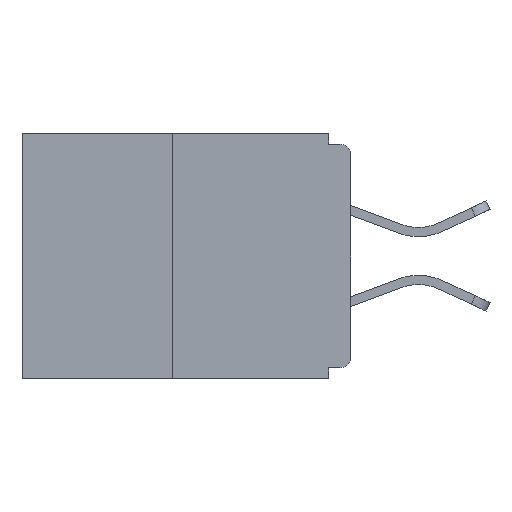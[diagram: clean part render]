
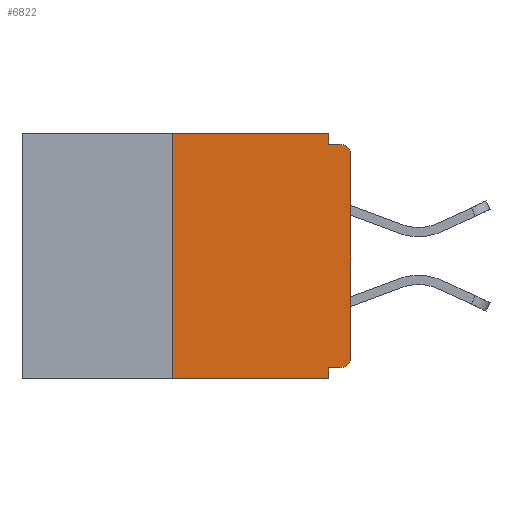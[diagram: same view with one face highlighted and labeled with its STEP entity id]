
A CAD part, left-side view. The second image highlights one B-rep face of the part: STEP entity #6822.
In plain terms, the highlighted planar face has unit normal (-1, 0, 0).
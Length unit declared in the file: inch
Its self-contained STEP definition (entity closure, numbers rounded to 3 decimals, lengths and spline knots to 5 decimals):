
#1 = CARTESIAN_POINT ( 'NONE',  ( 0., 0.25, -0.343 ) ) ;
#518 = LINE ( 'NONE', #16993, #8236 ) ;
#645 = CIRCLE ( 'NONE', #3352, 0.015 ) ;
#702 = VERTEX_POINT ( 'NONE', #1 ) ;
#794 = VERTEX_POINT ( 'NONE', #14768 ) ;
#949 = DIRECTION ( 'NONE',  ( 0., 0., 1. ) ) ;
#1246 = DIRECTION ( 'NONE',  ( -1., 0., 0. ) ) ;
#1406 = ORIENTED_EDGE ( 'NONE', *, *, #11811, .T. ) ;
#2094 = EDGE_CURVE ( 'NONE', #702, #5906, #8953, .T. ) ;
#2279 = AXIS2_PLACEMENT_3D ( 'NONE', #16837, #4396, #8564 ) ;
#2328 = CARTESIAN_POINT ( 'NONE',  ( 0., 0.015, -0.328 ) ) ;
#2385 = VECTOR ( 'NONE', #15722, 39.37008 ) ;
#2695 = EDGE_CURVE ( 'NONE', #12157, #14163, #15593, .T. ) ;
#2915 = AXIS2_PLACEMENT_3D ( 'NONE', #4314, #13677, #6977 ) ;
#3200 = CARTESIAN_POINT ( 'NONE',  ( 0., 0.031, -0.343 ) ) ;
#3352 = AXIS2_PLACEMENT_3D ( 'NONE', #9292, #1246, #3997 ) ;
#3431 = EDGE_CURVE ( 'NONE', #702, #12221, #518, .T. ) ;
#3576 = DIRECTION ( 'NONE',  ( 0., -1., 0. ) ) ;
#3997 = DIRECTION ( 'NONE',  ( 0., 0., -1. ) ) ;
#4223 = CARTESIAN_POINT ( 'NONE',  ( 0., 0., -0.313 ) ) ;
#4314 = CARTESIAN_POINT ( 'NONE',  ( 0., 0.015, -0.03 ) ) ;
#4396 = DIRECTION ( 'NONE',  ( 1., 0., 0. ) ) ;
#4403 = CARTESIAN_POINT ( 'NONE',  ( 0., 0.46, -0.343 ) ) ;
#4860 = CARTESIAN_POINT ( 'NONE',  ( 0., 0.031, -0.343 ) ) ;
#5455 = ORIENTED_EDGE ( 'NONE', *, *, #3431, .F. ) ;
#5906 = VERTEX_POINT ( 'NONE', #3200 ) ;
#6229 = EDGE_CURVE ( 'NONE', #12221, #12157, #12163, .T. ) ;
#6442 = DIRECTION ( 'NONE',  ( 0., 1., 0. ) ) ;
#6633 = VECTOR ( 'NONE', #7655, 39.37008 ) ;
#6822 = ADVANCED_FACE ( 'NONE', ( #11078 ), #9447, .F. ) ;
#6977 = DIRECTION ( 'NONE',  ( 0., 0., -1. ) ) ;
#7655 = DIRECTION ( 'NONE',  ( 0., 0., -1. ) ) ;
#7706 = DIRECTION ( 'NONE',  ( 0., 0., 1. ) ) ;
#8236 = VECTOR ( 'NONE', #7706, 39.37008 ) ;
#8486 = EDGE_CURVE ( 'NONE', #11581, #794, #11215, .T. ) ;
#8564 = DIRECTION ( 'NONE',  ( 0., 0., -1. ) ) ;
#8953 = LINE ( 'NONE', #4403, #14776 ) ;
#9248 = CARTESIAN_POINT ( 'NONE',  ( 0., 0.031, 0. ) ) ;
#9292 = CARTESIAN_POINT ( 'NONE',  ( 0., 0.015, -0.313 ) ) ;
#9447 = PLANE ( 'NONE',  #2279 ) ;
#9465 = DIRECTION ( 'NONE',  ( 0., -1., 0. ) ) ;
#9613 = EDGE_CURVE ( 'NONE', #14163, #11560, #16160, .T. ) ;
#9620 = CARTESIAN_POINT ( 'NONE',  ( 0., 0.015, -0.015 ) ) ;
#10365 = VECTOR ( 'NONE', #949, 39.37008 ) ;
#10886 = CARTESIAN_POINT ( 'NONE',  ( 0., 0.46, 0. ) ) ;
#10889 = EDGE_CURVE ( 'NONE', #13021, #11581, #645, .T. ) ;
#10909 = EDGE_LOOP ( 'NONE', ( #13129, #5455, #15306, #12876, #14455, #11340, #14215, #1406, #14113, #12107 ) ) ;
#11078 = FACE_OUTER_BOUND ( 'NONE', #10909, .T. ) ;
#11215 = LINE ( 'NONE', #15340, #10365 ) ;
#11340 = ORIENTED_EDGE ( 'NONE', *, *, #10889, .T. ) ;
#11560 = VERTEX_POINT ( 'NONE', #9620 ) ;
#11581 = VERTEX_POINT ( 'NONE', #4223 ) ;
#11635 = CARTESIAN_POINT ( 'NONE',  ( 0., 0., -0.015 ) ) ;
#11811 = EDGE_CURVE ( 'NONE', #794, #11560, #13368, .T. ) ;
#12107 = ORIENTED_EDGE ( 'NONE', *, *, #2695, .F. ) ;
#12157 = VERTEX_POINT ( 'NONE', #9248 ) ;
#12163 = LINE ( 'NONE', #10886, #17300 ) ;
#12221 = VERTEX_POINT ( 'NONE', #13739 ) ;
#12876 = ORIENTED_EDGE ( 'NONE', *, *, #13580, .F. ) ;
#13021 = VERTEX_POINT ( 'NONE', #2328 ) ;
#13036 = EDGE_CURVE ( 'NONE', #13021, #13071, #16088, .T. ) ;
#13071 = VERTEX_POINT ( 'NONE', #13077 ) ;
#13077 = CARTESIAN_POINT ( 'NONE',  ( 0., 0.031, -0.328 ) ) ;
#13129 = ORIENTED_EDGE ( 'NONE', *, *, #6229, .F. ) ;
#13368 = CIRCLE ( 'NONE', #2915, 0.015 ) ;
#13580 = EDGE_CURVE ( 'NONE', #13071, #5906, #16478, .T. ) ;
#13677 = DIRECTION ( 'NONE',  ( -1., 0., 0. ) ) ;
#13693 = CARTESIAN_POINT ( 'NONE',  ( 0., 0.031, -0.015 ) ) ;
#13739 = CARTESIAN_POINT ( 'NONE',  ( 0., 0.25, 0. ) ) ;
#14004 = VECTOR ( 'NONE', #6442, 39.37008 ) ;
#14113 = ORIENTED_EDGE ( 'NONE', *, *, #9613, .F. ) ;
#14163 = VERTEX_POINT ( 'NONE', #13693 ) ;
#14215 = ORIENTED_EDGE ( 'NONE', *, *, #8486, .T. ) ;
#14431 = CARTESIAN_POINT ( 'NONE',  ( 0., 0.031, 0. ) ) ;
#14455 = ORIENTED_EDGE ( 'NONE', *, *, #13036, .F. ) ;
#14768 = CARTESIAN_POINT ( 'NONE',  ( 0., 0., -0.03 ) ) ;
#14776 = VECTOR ( 'NONE', #16550, 39.37008 ) ;
#15132 = VECTOR ( 'NONE', #3576, 39.37008 ) ;
#15306 = ORIENTED_EDGE ( 'NONE', *, *, #2094, .T. ) ;
#15340 = CARTESIAN_POINT ( 'NONE',  ( 0., 0., 0. ) ) ;
#15593 = LINE ( 'NONE', #14431, #2385 ) ;
#15722 = DIRECTION ( 'NONE',  ( 0., 0., -1. ) ) ;
#16088 = LINE ( 'NONE', #16905, #14004 ) ;
#16160 = LINE ( 'NONE', #11635, #15132 ) ;
#16478 = LINE ( 'NONE', #4860, #6633 ) ;
#16550 = DIRECTION ( 'NONE',  ( 0., -1., 0. ) ) ;
#16837 = CARTESIAN_POINT ( 'NONE',  ( 0., 0.46, 0. ) ) ;
#16905 = CARTESIAN_POINT ( 'NONE',  ( 0., 0., -0.328 ) ) ;
#16993 = CARTESIAN_POINT ( 'NONE',  ( 0., 0.25, 0. ) ) ;
#17300 = VECTOR ( 'NONE', #9465, 39.37008 ) ;
